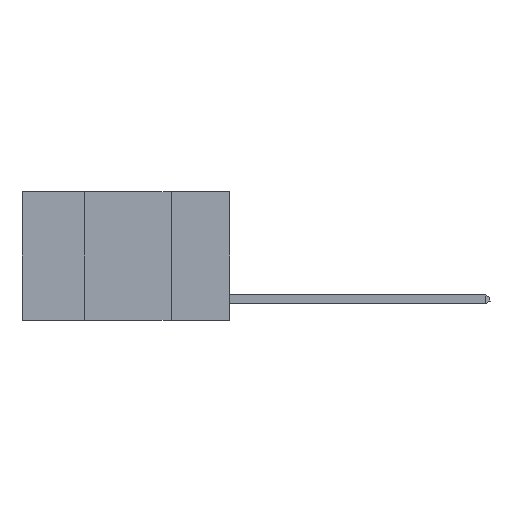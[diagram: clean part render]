
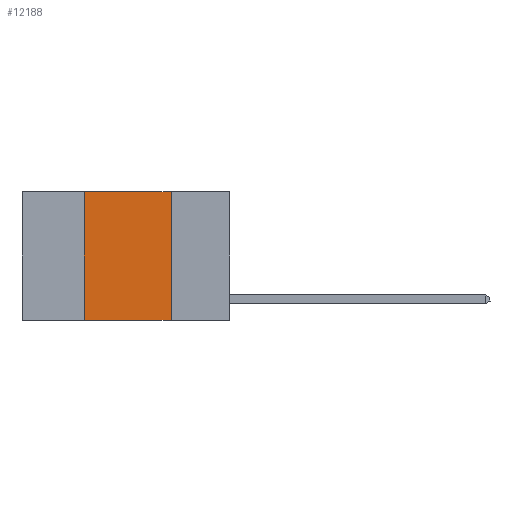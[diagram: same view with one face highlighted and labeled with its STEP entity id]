
A CAD part, left-side view. The second image highlights one B-rep face of the part: STEP entity #12188.
In plain terms, the highlighted planar face has unit normal (-1, 0, 0).
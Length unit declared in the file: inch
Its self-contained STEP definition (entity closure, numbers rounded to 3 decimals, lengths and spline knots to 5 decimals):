
#607 = EDGE_CURVE ( 'NONE', #1942, #19561, #3642, .T. ) ;
#1715 = VERTEX_POINT ( 'NONE', #3503 ) ;
#1942 = VERTEX_POINT ( 'NONE', #11633 ) ;
#1994 = EDGE_CURVE ( 'NONE', #8058, #1942, #19191, .T. ) ;
#2432 = VECTOR ( 'NONE', #9820, 39.37008 ) ;
#2622 = DIRECTION ( 'NONE',  ( 0., 0., 1. ) ) ;
#3503 = CARTESIAN_POINT ( 'NONE',  ( 0., 0.17, -0.37 ) ) ;
#3642 = LINE ( 'NONE', #4134, #8212 ) ;
#3669 = CARTESIAN_POINT ( 'NONE',  ( 0., 0.6, 0. ) ) ;
#4036 = ORIENTED_EDGE ( 'NONE', *, *, #12208, .F. ) ;
#4134 = CARTESIAN_POINT ( 'NONE',  ( 0., 0.6, 0. ) ) ;
#4567 = DIRECTION ( 'NONE',  ( 0., -1., 0. ) ) ;
#5199 = DIRECTION ( 'NONE',  ( 0., 0., -1. ) ) ;
#5826 = LINE ( 'NONE', #19159, #17902 ) ;
#6744 = CARTESIAN_POINT ( 'NONE',  ( 0., 0.17, 0. ) ) ;
#7447 = LINE ( 'NONE', #6744, #2432 ) ;
#8058 = VERTEX_POINT ( 'NONE', #12287 ) ;
#8212 = VECTOR ( 'NONE', #4567, 39.37008 ) ;
#9820 = DIRECTION ( 'NONE',  ( 0., 0., -1. ) ) ;
#10242 = CARTESIAN_POINT ( 'NONE',  ( 0., 0.42, 0. ) ) ;
#10554 = FACE_OUTER_BOUND ( 'NONE', #18614, .T. ) ;
#11283 = PLANE ( 'NONE',  #15814 ) ;
#11633 = CARTESIAN_POINT ( 'NONE',  ( 0., 0.42, 0. ) ) ;
#11709 = DIRECTION ( 'NONE',  ( 0., -1., 0. ) ) ;
#12188 = ADVANCED_FACE ( 'NONE', ( #10554 ), #11283, .F. ) ;
#12208 = EDGE_CURVE ( 'NONE', #19561, #1715, #7447, .T. ) ;
#12287 = CARTESIAN_POINT ( 'NONE',  ( 0., 0.42, -0.37 ) ) ;
#13094 = ORIENTED_EDGE ( 'NONE', *, *, #607, .F. ) ;
#13564 = ORIENTED_EDGE ( 'NONE', *, *, #1994, .F. ) ;
#14025 = ORIENTED_EDGE ( 'NONE', *, *, #18602, .T. ) ;
#14297 = DIRECTION ( 'NONE',  ( 1., 0., 0. ) ) ;
#15211 = VECTOR ( 'NONE', #2622, 39.37008 ) ;
#15814 = AXIS2_PLACEMENT_3D ( 'NONE', #3669, #14297, #5199 ) ;
#17902 = VECTOR ( 'NONE', #11709, 39.37008 ) ;
#18413 = CARTESIAN_POINT ( 'NONE',  ( 0., 0.17, 0. ) ) ;
#18602 = EDGE_CURVE ( 'NONE', #8058, #1715, #5826, .T. ) ;
#18614 = EDGE_LOOP ( 'NONE', ( #4036, #13094, #13564, #14025 ) ) ;
#19159 = CARTESIAN_POINT ( 'NONE',  ( 0., 0.6, -0.37 ) ) ;
#19191 = LINE ( 'NONE', #10242, #15211 ) ;
#19561 = VERTEX_POINT ( 'NONE', #18413 ) ;
